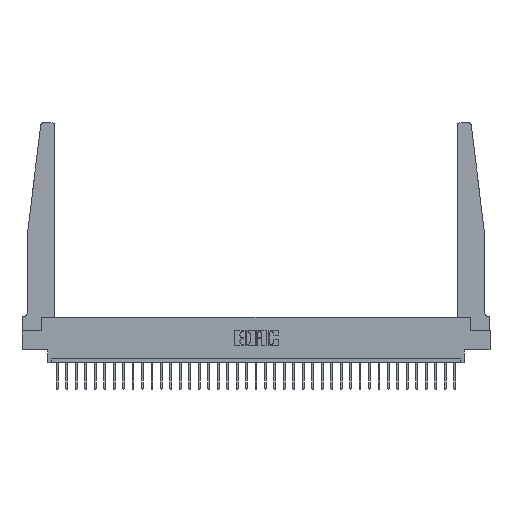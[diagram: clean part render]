
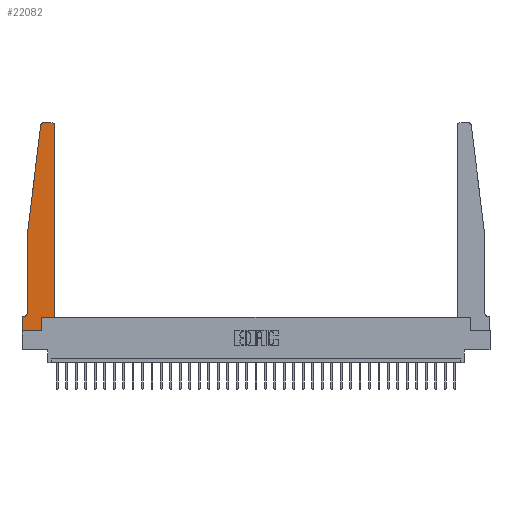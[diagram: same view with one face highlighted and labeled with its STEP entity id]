
A CAD part, top view. The second image highlights one B-rep face of the part: STEP entity #22082.
In plain terms, the highlighted planar face has unit normal (0, 0, 1).
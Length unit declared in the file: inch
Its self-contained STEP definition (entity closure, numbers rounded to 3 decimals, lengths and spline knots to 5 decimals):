
#284 = CARTESIAN_POINT ( 'NONE',  ( 0., 0., 0.37 ) ) ;
#490 = VECTOR ( 'NONE', #18560, 39.37008 ) ;
#883 = ORIENTED_EDGE ( 'NONE', *, *, #28979, .T. ) ;
#1337 = DIRECTION ( 'NONE',  ( -1., 0., 0. ) ) ;
#1593 = CARTESIAN_POINT ( 'NONE',  ( 0.27653, 2.72, 0.37 ) ) ;
#1636 = ORIENTED_EDGE ( 'NONE', *, *, #20969, .T. ) ;
#2177 = VECTOR ( 'NONE', #19402, 39.37008 ) ;
#2410 = AXIS2_PLACEMENT_3D ( 'NONE', #25088, #27372, #27681 ) ;
#2414 = DIRECTION ( 'NONE',  ( -1., 0., 0. ) ) ;
#2490 = LINE ( 'NONE', #4434, #490 ) ;
#2547 = LINE ( 'NONE', #15286, #25314 ) ;
#2660 = EDGE_CURVE ( 'NONE', #20190, #26035, #2547, .T. ) ;
#3001 = CARTESIAN_POINT ( 'NONE',  ( 0.2605, 0.18, 0.37 ) ) ;
#3883 = DIRECTION ( 'NONE',  ( 1., 0., 0. ) ) ;
#3984 = DIRECTION ( 'NONE',  ( -1., 0., 0. ) ) ;
#4027 = DIRECTION ( 'NONE',  ( 0., 0., 1. ) ) ;
#4312 = CARTESIAN_POINT ( 'NONE',  ( 0.065, 1.25, 0.37 ) ) ;
#4327 = CARTESIAN_POINT ( 'NONE',  ( 0.425, 2.72, 0.37 ) ) ;
#4434 = CARTESIAN_POINT ( 'NONE',  ( 0.065, 1.25, 0.37 ) ) ;
#4724 = AXIS2_PLACEMENT_3D ( 'NONE', #1593, #4027, #11405 ) ;
#4738 = LINE ( 'NONE', #9813, #22229 ) ;
#4741 = ORIENTED_EDGE ( 'NONE', *, *, #2660, .T. ) ;
#4743 = DIRECTION ( 'NONE',  ( 0., 0., -1. ) ) ;
#4922 = VERTEX_POINT ( 'NONE', #3001 ) ;
#5483 = EDGE_LOOP ( 'NONE', ( #30216, #12251, #883, #26955, #27543, #27116, #30665, #4741, #1636, #10080, #12049, #17131 ) ) ;
#5798 = VERTEX_POINT ( 'NONE', #22188 ) ;
#6536 = EDGE_CURVE ( 'NONE', #4922, #29052, #13507, .T. ) ;
#6641 = VECTOR ( 'NONE', #28364, 39.37008 ) ;
#7218 = CARTESIAN_POINT ( 'NONE',  ( 0.425, 0.18, 0.37 ) ) ;
#7839 = CARTESIAN_POINT ( 'NONE',  ( 0.015, 0.1875, 0.37 ) ) ;
#7923 = EDGE_CURVE ( 'NONE', #25596, #28810, #9724, .T. ) ;
#8564 = EDGE_CURVE ( 'NONE', #20919, #20190, #4738, .T. ) ;
#9032 = VERTEX_POINT ( 'NONE', #10320 ) ;
#9260 = CIRCLE ( 'NONE', #2410, 0.03 ) ;
#9724 = CIRCLE ( 'NONE', #4724, 0.03 ) ;
#9813 = CARTESIAN_POINT ( 'NONE',  ( 0., 0., 0.37 ) ) ;
#10080 = ORIENTED_EDGE ( 'NONE', *, *, #6536, .T. ) ;
#10320 = CARTESIAN_POINT ( 'NONE',  ( 0.395, 2.75, 0.37 ) ) ;
#10807 = DIRECTION ( 'NONE',  ( 0., 0., 1. ) ) ;
#11405 = DIRECTION ( 'NONE',  ( 1., 0., 0. ) ) ;
#11441 = VECTOR ( 'NONE', #1337, 39.37008 ) ;
#12049 = ORIENTED_EDGE ( 'NONE', *, *, #27405, .T. ) ;
#12251 = ORIENTED_EDGE ( 'NONE', *, *, #7923, .T. ) ;
#12636 = LINE ( 'NONE', #21197, #6641 ) ;
#12823 = DIRECTION ( 'NONE',  ( 0., 1., 0. ) ) ;
#12955 = EDGE_CURVE ( 'NONE', #19916, #5798, #18095, .T. ) ;
#13507 = LINE ( 'NONE', #7218, #2177 ) ;
#14328 = CARTESIAN_POINT ( 'NONE',  ( 0.015, 0.2375, 0.37 ) ) ;
#14663 = EDGE_CURVE ( 'NONE', #5798, #29244, #20279, .T. ) ;
#14726 = AXIS2_PLACEMENT_3D ( 'NONE', #25264, #10807, #27965 ) ;
#15286 = CARTESIAN_POINT ( 'NONE',  ( 0., 0., 0.37 ) ) ;
#15758 = CARTESIAN_POINT ( 'NONE',  ( 0.24675, 2.72367, 0.37 ) ) ;
#15925 = LINE ( 'NONE', #26086, #25078 ) ;
#16373 = DIRECTION ( 'NONE',  ( 0., -1., 0. ) ) ;
#16607 = CARTESIAN_POINT ( 'NONE',  ( 0.425, 0.18, 0.37 ) ) ;
#17097 = CARTESIAN_POINT ( 'NONE',  ( 0.27653, 2.75, 0.37 ) ) ;
#17131 = ORIENTED_EDGE ( 'NONE', *, *, #21432, .T. ) ;
#17664 = EDGE_CURVE ( 'NONE', #29244, #20919, #15925, .T. ) ;
#18095 = LINE ( 'NONE', #26116, #27665 ) ;
#18126 = VERTEX_POINT ( 'NONE', #4327 ) ;
#18560 = DIRECTION ( 'NONE',  ( -0.122, -0.992, 0. ) ) ;
#18583 = EDGE_CURVE ( 'NONE', #9032, #25596, #28493, .T. ) ;
#19402 = DIRECTION ( 'NONE',  ( 1., 0., 0. ) ) ;
#19916 = VERTEX_POINT ( 'NONE', #4312 ) ;
#20190 = VERTEX_POINT ( 'NONE', #284 ) ;
#20279 = CIRCLE ( 'NONE', #20582, 0.05 ) ;
#20582 = AXIS2_PLACEMENT_3D ( 'NONE', #14328, #4743, #2414 ) ;
#20919 = VERTEX_POINT ( 'NONE', #27933 ) ;
#20969 = EDGE_CURVE ( 'NONE', #26035, #4922, #12636, .T. ) ;
#21197 = CARTESIAN_POINT ( 'NONE',  ( 0.2605, 0.18, 0.37 ) ) ;
#21432 = EDGE_CURVE ( 'NONE', #18126, #9032, #9260, .T. ) ;
#21574 = CARTESIAN_POINT ( 'NONE',  ( 0.2605, 0., 0.37 ) ) ;
#21594 = LINE ( 'NONE', #30032, #26556 ) ;
#22082 = ADVANCED_FACE ( 'NONE', ( #27878 ), #22939, .T. ) ;
#22188 = CARTESIAN_POINT ( 'NONE',  ( 0.065, 0.2375, 0.37 ) ) ;
#22229 = VECTOR ( 'NONE', #22244, 39.37008 ) ;
#22244 = DIRECTION ( 'NONE',  ( 0., -1., 0. ) ) ;
#22784 = CARTESIAN_POINT ( 'NONE',  ( 0.25, 2.75, 0.37 ) ) ;
#22939 = PLANE ( 'NONE',  #14726 ) ;
#25078 = VECTOR ( 'NONE', #3984, 39.37008 ) ;
#25088 = CARTESIAN_POINT ( 'NONE',  ( 0.395, 2.72, 0.37 ) ) ;
#25264 = CARTESIAN_POINT ( 'NONE',  ( 0., 0.1875, 0.37 ) ) ;
#25314 = VECTOR ( 'NONE', #3883, 39.37008 ) ;
#25596 = VERTEX_POINT ( 'NONE', #17097 ) ;
#26035 = VERTEX_POINT ( 'NONE', #21574 ) ;
#26086 = CARTESIAN_POINT ( 'NONE',  ( 0.065, 0.1875, 0.37 ) ) ;
#26116 = CARTESIAN_POINT ( 'NONE',  ( 0.065, 1.25, 0.37 ) ) ;
#26556 = VECTOR ( 'NONE', #12823, 39.37008 ) ;
#26955 = ORIENTED_EDGE ( 'NONE', *, *, #12955, .T. ) ;
#27116 = ORIENTED_EDGE ( 'NONE', *, *, #17664, .T. ) ;
#27372 = DIRECTION ( 'NONE',  ( 0., 0., 1. ) ) ;
#27405 = EDGE_CURVE ( 'NONE', #29052, #18126, #21594, .T. ) ;
#27543 = ORIENTED_EDGE ( 'NONE', *, *, #14663, .T. ) ;
#27665 = VECTOR ( 'NONE', #16373, 39.37008 ) ;
#27681 = DIRECTION ( 'NONE',  ( 1., 0., 0. ) ) ;
#27878 = FACE_OUTER_BOUND ( 'NONE', #5483, .T. ) ;
#27933 = CARTESIAN_POINT ( 'NONE',  ( 0., 0.1875, 0.37 ) ) ;
#27965 = DIRECTION ( 'NONE',  ( 1., 0., 0. ) ) ;
#28364 = DIRECTION ( 'NONE',  ( 0., 1., 0. ) ) ;
#28493 = LINE ( 'NONE', #22784, #11441 ) ;
#28810 = VERTEX_POINT ( 'NONE', #15758 ) ;
#28979 = EDGE_CURVE ( 'NONE', #28810, #19916, #2490, .T. ) ;
#29052 = VERTEX_POINT ( 'NONE', #16607 ) ;
#29244 = VERTEX_POINT ( 'NONE', #7839 ) ;
#30032 = CARTESIAN_POINT ( 'NONE',  ( 0.425, 0.18, 0.37 ) ) ;
#30216 = ORIENTED_EDGE ( 'NONE', *, *, #18583, .T. ) ;
#30665 = ORIENTED_EDGE ( 'NONE', *, *, #8564, .T. ) ;
